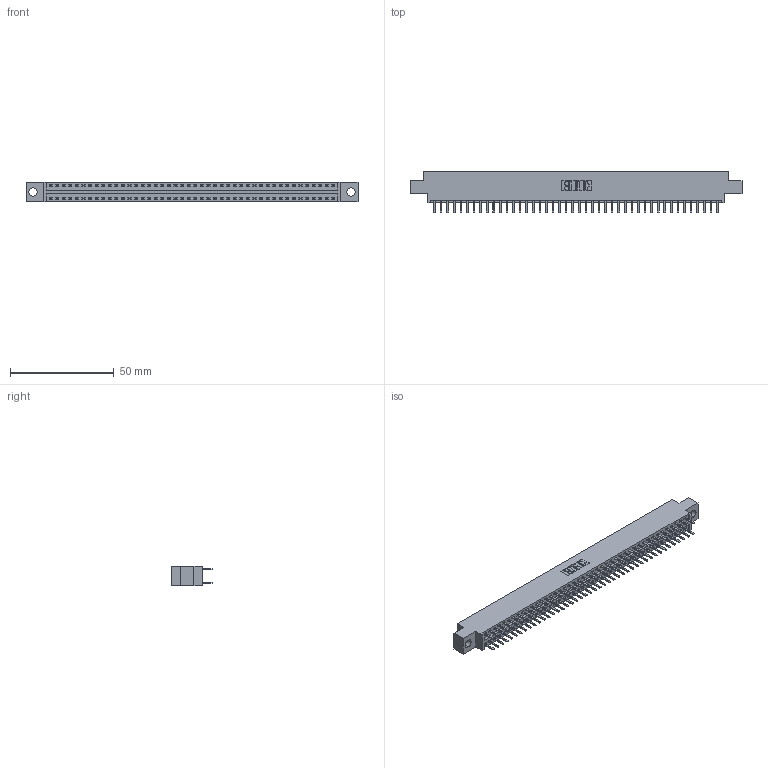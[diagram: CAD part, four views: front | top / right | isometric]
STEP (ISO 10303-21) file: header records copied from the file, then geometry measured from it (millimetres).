
FILE_DESCRIPTION (( 'STEP AP203' ), '1' );
FILE_NAME ('396-088-520-804.STEP', '2019-11-02T14:59:16', ( '' ), ( '' ), 'SwSTEP 2.0', 'SolidWorks 2016', '' );
FILE_SCHEMA (( 'CONFIG_CONTROL_DESIGN' ));
Length unit declared in the file: inch
Products named in the file (3): 346 Part_0.170 Offset - 0.156 Dia-TH; 345-292-001_345-293-120; 396-088-520-804
Assembly tree (89 placements, depth 2):
  396-088-520-804
    346 Part_0.170 Offset - 0.156 Dia-TH
    345-292-001_345-293-120  x88
Bounding box: 160.27 x 20.02 x 9.4 mm (x, y, z)
Volume: 15363.1 mm3; surface area: 21051.4 mm2
Topology: 89 solids, 89 shells, 5054 faces, 14685 edges, 9554 vertices
Faces by surface type: plane 3336, cylinder 1718
Entity records: 28695 total; most frequent: CARTESIAN_POINT 4740, ORIENTED_EDGE 4662, DIRECTION 4215, EDGE_CURVE 2331, LINE 2019, VECTOR 2019, VERTEX_POINT 1550, AXIS2_PLACEMENT_3D 1098
